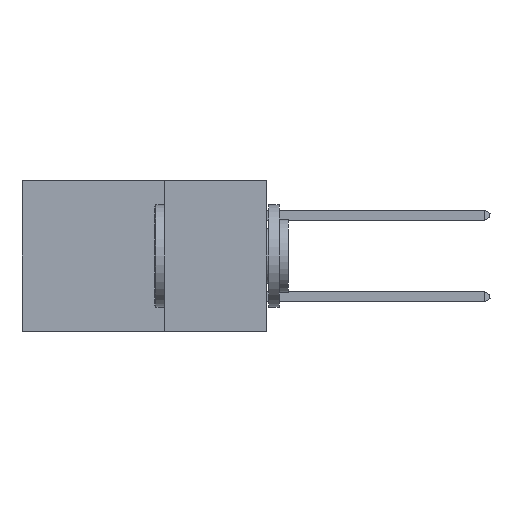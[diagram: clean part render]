
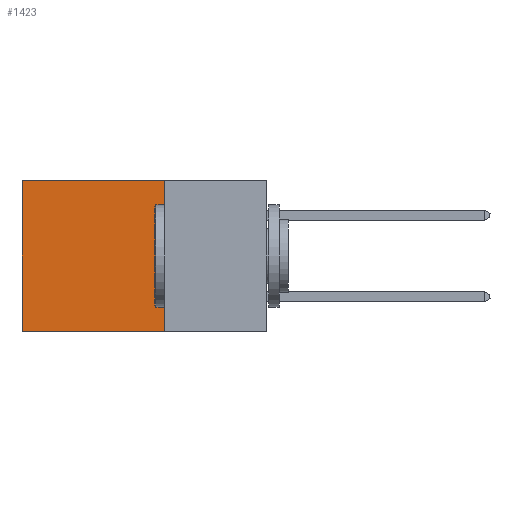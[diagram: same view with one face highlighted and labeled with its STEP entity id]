
A CAD part, left-side view. The second image highlights one B-rep face of the part: STEP entity #1423.
In plain terms, the highlighted planar face has unit normal (-1, 0, 0).
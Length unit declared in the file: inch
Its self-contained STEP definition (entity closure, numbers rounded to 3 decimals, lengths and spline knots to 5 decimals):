
#27 = VECTOR ( 'NONE', #20451, 39.37008 ) ;
#755 = CARTESIAN_POINT ( 'NONE',  ( 0.2875, 0.25, 0. ) ) ;
#819 = ORIENTED_EDGE ( 'NONE', *, *, #32065, .F. ) ;
#892 = VERTEX_POINT ( 'NONE', #15154 ) ;
#1423 = ADVANCED_FACE ( 'NONE', ( #25240 ), #30509, .F. ) ;
#2245 = EDGE_CURVE ( 'NONE', #24860, #892, #18267, .T. ) ;
#3150 = VECTOR ( 'NONE', #26013, 39.37008 ) ;
#5338 = VECTOR ( 'NONE', #12577, 39.37008 ) ;
#5962 = CARTESIAN_POINT ( 'NONE',  ( 0.2875, 0.25, 0. ) ) ;
#6557 = CARTESIAN_POINT ( 'NONE',  ( 0.2875, 0.25, 0. ) ) ;
#7680 = VERTEX_POINT ( 'NONE', #26715 ) ;
#8230 = DIRECTION ( 'NONE',  ( 0., 1., 0. ) ) ;
#11241 = CARTESIAN_POINT ( 'NONE',  ( 0.2875, 0.25, -0.37 ) ) ;
#12577 = DIRECTION ( 'NONE',  ( 0., 0., -1. ) ) ;
#14262 = DIRECTION ( 'NONE',  ( 0., 0., -1. ) ) ;
#14307 = EDGE_CURVE ( 'NONE', #7680, #24860, #16893, .T. ) ;
#14937 = VECTOR ( 'NONE', #8230, 39.37008 ) ;
#15154 = CARTESIAN_POINT ( 'NONE',  ( 0.2875, 0.6, -0.37 ) ) ;
#16893 = LINE ( 'NONE', #755, #3150 ) ;
#16982 = AXIS2_PLACEMENT_3D ( 'NONE', #5962, #28004, #14262 ) ;
#17464 = EDGE_CURVE ( 'NONE', #24247, #892, #22294, .T. ) ;
#18267 = LINE ( 'NONE', #21145, #5338 ) ;
#18308 = ORIENTED_EDGE ( 'NONE', *, *, #17464, .F. ) ;
#20451 = DIRECTION ( 'NONE',  ( 0., 0., -1. ) ) ;
#21145 = CARTESIAN_POINT ( 'NONE',  ( 0.2875, 0.6, 0. ) ) ;
#22294 = LINE ( 'NONE', #11241, #14937 ) ;
#24247 = VERTEX_POINT ( 'NONE', #32660 ) ;
#24860 = VERTEX_POINT ( 'NONE', #31761 ) ;
#25165 = EDGE_LOOP ( 'NONE', ( #31334, #18308, #819, #27107 ) ) ;
#25240 = FACE_OUTER_BOUND ( 'NONE', #25165, .T. ) ;
#26013 = DIRECTION ( 'NONE',  ( 0., 1., 0. ) ) ;
#26715 = CARTESIAN_POINT ( 'NONE',  ( 0.2875, 0.25, 0. ) ) ;
#27107 = ORIENTED_EDGE ( 'NONE', *, *, #14307, .T. ) ;
#28004 = DIRECTION ( 'NONE',  ( 1., 0., 0. ) ) ;
#30509 = PLANE ( 'NONE',  #16982 ) ;
#31334 = ORIENTED_EDGE ( 'NONE', *, *, #2245, .T. ) ;
#31398 = LINE ( 'NONE', #6557, #27 ) ;
#31761 = CARTESIAN_POINT ( 'NONE',  ( 0.2875, 0.6, 0. ) ) ;
#32065 = EDGE_CURVE ( 'NONE', #7680, #24247, #31398, .T. ) ;
#32660 = CARTESIAN_POINT ( 'NONE',  ( 0.2875, 0.25, -0.37 ) ) ;
